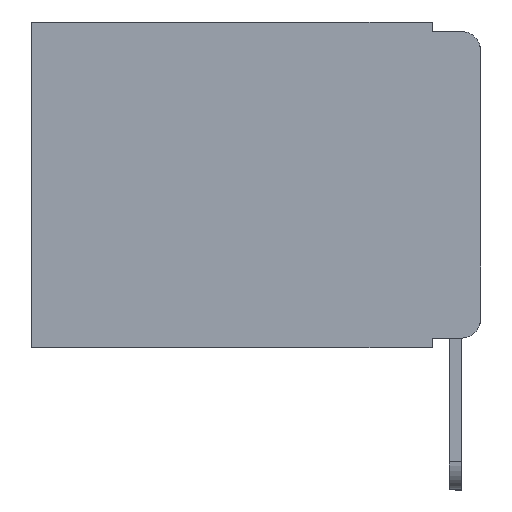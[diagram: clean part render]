
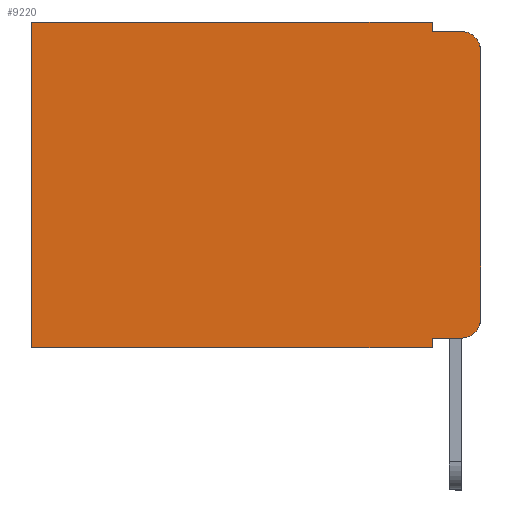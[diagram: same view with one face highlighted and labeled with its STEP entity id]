
A CAD part, left-side view. The second image highlights one B-rep face of the part: STEP entity #9220.
In plain terms, the highlighted planar face has unit normal (-1, 0, 0).
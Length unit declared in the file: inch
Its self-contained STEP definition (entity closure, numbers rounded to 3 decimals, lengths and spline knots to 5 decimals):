
#855 = VERTEX_POINT ( 'NONE', #2262 ) ;
#950 = ORIENTED_EDGE ( 'NONE', *, *, #24845, .F. ) ;
#1153 = EDGE_LOOP ( 'NONE', ( #950, #6057, #19738, #13531, #14634, #14695, #11861, #11188, #24312, #8022 ) ) ;
#2145 = LINE ( 'NONE', #21880, #18970 ) ;
#2262 = CARTESIAN_POINT ( 'NONE',  ( 0.298, 0.051, -0.333 ) ) ;
#2616 = CARTESIAN_POINT ( 'NONE',  ( 0.298, 0.473, 0. ) ) ;
#3131 = DIRECTION ( 'NONE',  ( -1., 0., 0. ) ) ;
#3770 = EDGE_CURVE ( 'NONE', #855, #15460, #21095, .T. ) ;
#4178 = CARTESIAN_POINT ( 'NONE',  ( 0.298, 0.02, -0.01 ) ) ;
#4442 = LINE ( 'NONE', #8755, #9651 ) ;
#4664 = CARTESIAN_POINT ( 'NONE',  ( 0.298, 0., -0.03 ) ) ;
#5063 = CARTESIAN_POINT ( 'NONE',  ( 0.298, 0.02, -0.313 ) ) ;
#5151 = AXIS2_PLACEMENT_3D ( 'NONE', #9366, #13517, #17262 ) ;
#5197 = EDGE_CURVE ( 'NONE', #855, #6663, #4442, .T. ) ;
#5918 = EDGE_CURVE ( 'NONE', #21026, #20808, #18357, .T. ) ;
#5983 = VECTOR ( 'NONE', #17441, 39.37008 ) ;
#6057 = ORIENTED_EDGE ( 'NONE', *, *, #5918, .T. ) ;
#6663 = VERTEX_POINT ( 'NONE', #10268 ) ;
#7039 = DIRECTION ( 'NONE',  ( 0., 1., 0. ) ) ;
#7249 = CARTESIAN_POINT ( 'NONE',  ( 0.298, 0.051, 0. ) ) ;
#7517 = CARTESIAN_POINT ( 'NONE',  ( 0.298, 0.473, 0. ) ) ;
#8022 = ORIENTED_EDGE ( 'NONE', *, *, #10979, .T. ) ;
#8755 = CARTESIAN_POINT ( 'NONE',  ( 0.298, 0.051, -0.333 ) ) ;
#8889 = DIRECTION ( 'NONE',  ( 0., 0., -1. ) ) ;
#9023 = EDGE_CURVE ( 'NONE', #15460, #18456, #17173, .T. ) ;
#9220 = ADVANCED_FACE ( 'NONE', ( #19093 ), #11569, .F. ) ;
#9366 = CARTESIAN_POINT ( 'NONE',  ( 0.298, 0., 0. ) ) ;
#9609 = DIRECTION ( 'NONE',  ( 0., 0., -1. ) ) ;
#9651 = VECTOR ( 'NONE', #20542, 39.37008 ) ;
#10204 = DIRECTION ( 'NONE',  ( 0., 0., -1. ) ) ;
#10268 = CARTESIAN_POINT ( 'NONE',  ( 0.298, 0.02, -0.333 ) ) ;
#10289 = EDGE_CURVE ( 'NONE', #21421, #12997, #11552, .T. ) ;
#10618 = VECTOR ( 'NONE', #9609, 39.37008 ) ;
#10979 = EDGE_CURVE ( 'NONE', #6663, #13422, #17697, .T. ) ;
#11076 = CARTESIAN_POINT ( 'NONE',  ( 0.298, 0., 0. ) ) ;
#11170 = CARTESIAN_POINT ( 'NONE',  ( 0.298, 0.473, -0.343 ) ) ;
#11188 = ORIENTED_EDGE ( 'NONE', *, *, #3770, .F. ) ;
#11552 = LINE ( 'NONE', #7249, #10618 ) ;
#11569 = PLANE ( 'NONE',  #5151 ) ;
#11861 = ORIENTED_EDGE ( 'NONE', *, *, #9023, .F. ) ;
#12905 = DIRECTION ( 'NONE',  ( -1., 0., 0. ) ) ;
#12997 = VERTEX_POINT ( 'NONE', #22041 ) ;
#13422 = VERTEX_POINT ( 'NONE', #25641 ) ;
#13517 = DIRECTION ( 'NONE',  ( 1., 0., 0. ) ) ;
#13531 = ORIENTED_EDGE ( 'NONE', *, *, #10289, .F. ) ;
#14144 = CARTESIAN_POINT ( 'NONE',  ( 0.298, 0.051, -0.343 ) ) ;
#14634 = ORIENTED_EDGE ( 'NONE', *, *, #16134, .T. ) ;
#14695 = ORIENTED_EDGE ( 'NONE', *, *, #19034, .T. ) ;
#15399 = VERTEX_POINT ( 'NONE', #7517 ) ;
#15460 = VERTEX_POINT ( 'NONE', #14144 ) ;
#15530 = CARTESIAN_POINT ( 'NONE',  ( 0.298, 0.051, 0. ) ) ;
#15876 = AXIS2_PLACEMENT_3D ( 'NONE', #18875, #12905, #8889 ) ;
#15971 = VECTOR ( 'NONE', #10204, 39.37008 ) ;
#16134 = EDGE_CURVE ( 'NONE', #21421, #15399, #18867, .T. ) ;
#17173 = LINE ( 'NONE', #20944, #5983 ) ;
#17222 = CARTESIAN_POINT ( 'NONE',  ( 0.298, 0., 0. ) ) ;
#17262 = DIRECTION ( 'NONE',  ( 0., 0., -1. ) ) ;
#17441 = DIRECTION ( 'NONE',  ( 0., 1., 0. ) ) ;
#17540 = DIRECTION ( 'NONE',  ( 0., 0., -1. ) ) ;
#17562 = VECTOR ( 'NONE', #7039, 39.37008 ) ;
#17697 = CIRCLE ( 'NONE', #19359, 0.02 ) ;
#18357 = CIRCLE ( 'NONE', #15876, 0.02 ) ;
#18456 = VERTEX_POINT ( 'NONE', #11170 ) ;
#18648 = DIRECTION ( 'NONE',  ( 0., 0., -1. ) ) ;
#18867 = LINE ( 'NONE', #11076, #17562 ) ;
#18875 = CARTESIAN_POINT ( 'NONE',  ( 0.298, 0.02, -0.03 ) ) ;
#18970 = VECTOR ( 'NONE', #22128, 39.37008 ) ;
#19034 = EDGE_CURVE ( 'NONE', #15399, #18456, #24085, .T. ) ;
#19093 = FACE_OUTER_BOUND ( 'NONE', #1153, .T. ) ;
#19359 = AXIS2_PLACEMENT_3D ( 'NONE', #5063, #3131, #17540 ) ;
#19738 = ORIENTED_EDGE ( 'NONE', *, *, #23333, .F. ) ;
#20542 = DIRECTION ( 'NONE',  ( 0., -1., 0. ) ) ;
#20808 = VERTEX_POINT ( 'NONE', #4178 ) ;
#20944 = CARTESIAN_POINT ( 'NONE',  ( 0.298, 0., -0.343 ) ) ;
#21026 = VERTEX_POINT ( 'NONE', #4664 ) ;
#21095 = LINE ( 'NONE', #24495, #22252 ) ;
#21421 = VERTEX_POINT ( 'NONE', #15530 ) ;
#21880 = CARTESIAN_POINT ( 'NONE',  ( 0.298, 0.051, -0.01 ) ) ;
#22041 = CARTESIAN_POINT ( 'NONE',  ( 0.298, 0.051, -0.01 ) ) ;
#22128 = DIRECTION ( 'NONE',  ( 0., -1., 0. ) ) ;
#22252 = VECTOR ( 'NONE', #18648, 39.37008 ) ;
#22927 = DIRECTION ( 'NONE',  ( 0., 0., -1. ) ) ;
#23333 = EDGE_CURVE ( 'NONE', #12997, #20808, #2145, .T. ) ;
#24085 = LINE ( 'NONE', #2616, #15971 ) ;
#24312 = ORIENTED_EDGE ( 'NONE', *, *, #5197, .T. ) ;
#24449 = VECTOR ( 'NONE', #22927, 39.37008 ) ;
#24495 = CARTESIAN_POINT ( 'NONE',  ( 0.298, 0.051, 0. ) ) ;
#24845 = EDGE_CURVE ( 'NONE', #21026, #13422, #24904, .T. ) ;
#24904 = LINE ( 'NONE', #17222, #24449 ) ;
#25641 = CARTESIAN_POINT ( 'NONE',  ( 0.298, 0., -0.313 ) ) ;
